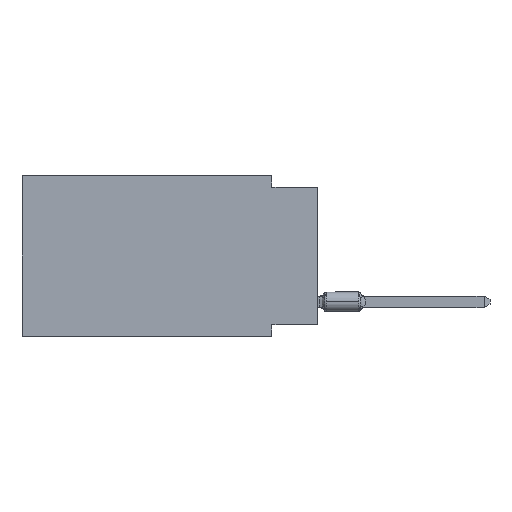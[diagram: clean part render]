
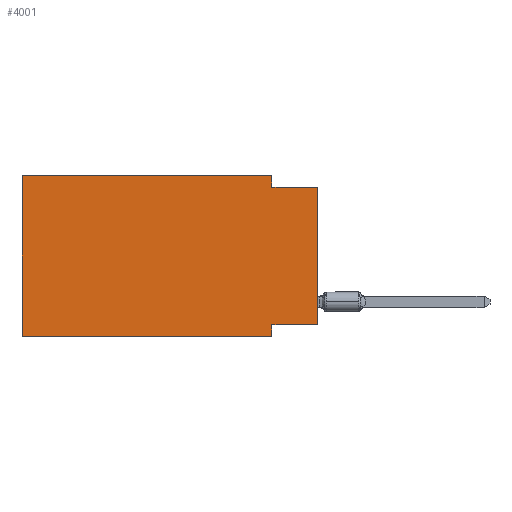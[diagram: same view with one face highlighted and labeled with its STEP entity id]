
A CAD part, left-side view. The second image highlights one B-rep face of the part: STEP entity #4001.
In plain terms, the highlighted planar face has unit normal (-1, 0, 0).
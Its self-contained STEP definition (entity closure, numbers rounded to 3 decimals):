
#301 = CARTESIAN_POINT ( 'NONE',  ( 0., 0., -8.255 ) ) ;
#351 = LINE ( 'NONE', #5917, #7434 ) ;
#478 = CARTESIAN_POINT ( 'NONE',  ( 0., 16.383, 0. ) ) ;
#701 = LINE ( 'NONE', #14898, #13395 ) ;
#754 = VECTOR ( 'NONE', #15659, 1000. ) ;
#1007 = CARTESIAN_POINT ( 'NONE',  ( 0., 16.383, 0. ) ) ;
#1133 = VECTOR ( 'NONE', #12843, 1000. ) ;
#1150 = DIRECTION ( 'NONE',  ( 0., -1., 0. ) ) ;
#1286 = CARTESIAN_POINT ( 'NONE',  ( 0., 0., -0.635 ) ) ;
#1605 = CARTESIAN_POINT ( 'NONE',  ( 0., 2.54, -8.255 ) ) ;
#1700 = CARTESIAN_POINT ( 'NONE',  ( 0., 2.54, -8.89 ) ) ;
#1791 = DIRECTION ( 'NONE',  ( 0., -1., 0. ) ) ;
#2219 = VECTOR ( 'NONE', #1791, 1000. ) ;
#2602 = ORIENTED_EDGE ( 'NONE', *, *, #8361, .T. ) ;
#2724 = VERTEX_POINT ( 'NONE', #1286 ) ;
#3174 = DIRECTION ( 'NONE',  ( 0., 0., -1. ) ) ;
#3936 = VERTEX_POINT ( 'NONE', #14567 ) ;
#4001 = ADVANCED_FACE ( 'NONE', ( #13475 ), #10969, .F. ) ;
#4195 = ORIENTED_EDGE ( 'NONE', *, *, #8038, .F. ) ;
#4328 = VECTOR ( 'NONE', #1150, 1000. ) ;
#4363 = VERTEX_POINT ( 'NONE', #7574 ) ;
#4878 = ORIENTED_EDGE ( 'NONE', *, *, #8454, .F. ) ;
#5448 = VERTEX_POINT ( 'NONE', #8599 ) ;
#5638 = LINE ( 'NONE', #8760, #2219 ) ;
#5833 = VERTEX_POINT ( 'NONE', #1605 ) ;
#5917 = CARTESIAN_POINT ( 'NONE',  ( 0., 16.383, 0. ) ) ;
#5918 = EDGE_LOOP ( 'NONE', ( #13003, #4195, #8770, #11957, #4878, #2602, #10950, #8723 ) ) ;
#6533 = LINE ( 'NONE', #10759, #4328 ) ;
#7222 = EDGE_CURVE ( 'NONE', #3936, #5833, #9633, .T. ) ;
#7434 = VECTOR ( 'NONE', #11496, 1000. ) ;
#7574 = CARTESIAN_POINT ( 'NONE',  ( 0., 2.54, 0. ) ) ;
#8038 = EDGE_CURVE ( 'NONE', #9749, #2724, #5638, .T. ) ;
#8113 = VERTEX_POINT ( 'NONE', #15612 ) ;
#8202 = VECTOR ( 'NONE', #12133, 1000. ) ;
#8361 = EDGE_CURVE ( 'NONE', #8113, #10505, #6533, .T. ) ;
#8454 = EDGE_CURVE ( 'NONE', #8113, #5448, #14306, .T. ) ;
#8599 = CARTESIAN_POINT ( 'NONE',  ( 0., 16.383, 0. ) ) ;
#8723 = ORIENTED_EDGE ( 'NONE', *, *, #7222, .F. ) ;
#8760 = CARTESIAN_POINT ( 'NONE',  ( 0., 0., -0.635 ) ) ;
#8770 = ORIENTED_EDGE ( 'NONE', *, *, #16653, .F. ) ;
#8938 = DIRECTION ( 'NONE',  ( 0., 0., 1. ) ) ;
#9289 = EDGE_CURVE ( 'NONE', #5448, #4363, #351, .T. ) ;
#9314 = EDGE_CURVE ( 'NONE', #5833, #10505, #15708, .T. ) ;
#9479 = CARTESIAN_POINT ( 'NONE',  ( 0., 2.54, 0. ) ) ;
#9633 = LINE ( 'NONE', #301, #754 ) ;
#9749 = VERTEX_POINT ( 'NONE', #10288 ) ;
#10288 = CARTESIAN_POINT ( 'NONE',  ( 0., 2.54, -0.635 ) ) ;
#10505 = VERTEX_POINT ( 'NONE', #1700 ) ;
#10759 = CARTESIAN_POINT ( 'NONE',  ( 0., 16.383, -8.89 ) ) ;
#10950 = ORIENTED_EDGE ( 'NONE', *, *, #9314, .F. ) ;
#10969 = PLANE ( 'NONE',  #17941 ) ;
#11226 = CARTESIAN_POINT ( 'NONE',  ( 0., 2.54, -8.89 ) ) ;
#11496 = DIRECTION ( 'NONE',  ( 0., -1., 0. ) ) ;
#11836 = EDGE_CURVE ( 'NONE', #3936, #2724, #701, .T. ) ;
#11957 = ORIENTED_EDGE ( 'NONE', *, *, #9289, .F. ) ;
#12133 = DIRECTION ( 'NONE',  ( 0., 0., -1. ) ) ;
#12355 = DIRECTION ( 'NONE',  ( 0., 0., -1. ) ) ;
#12843 = DIRECTION ( 'NONE',  ( 0., 0., 1. ) ) ;
#13003 = ORIENTED_EDGE ( 'NONE', *, *, #11836, .T. ) ;
#13395 = VECTOR ( 'NONE', #8938, 1000. ) ;
#13475 = FACE_OUTER_BOUND ( 'NONE', #5918, .T. ) ;
#13710 = LINE ( 'NONE', #9479, #8202 ) ;
#14306 = LINE ( 'NONE', #478, #1133 ) ;
#14567 = CARTESIAN_POINT ( 'NONE',  ( 0., 0., -8.255 ) ) ;
#14748 = DIRECTION ( 'NONE',  ( 1., 0., 0. ) ) ;
#14898 = CARTESIAN_POINT ( 'NONE',  ( 0., 0., 0. ) ) ;
#15612 = CARTESIAN_POINT ( 'NONE',  ( 0., 16.383, -8.89 ) ) ;
#15659 = DIRECTION ( 'NONE',  ( 0., 1., 0. ) ) ;
#15708 = LINE ( 'NONE', #11226, #17692 ) ;
#16653 = EDGE_CURVE ( 'NONE', #4363, #9749, #13710, .T. ) ;
#17692 = VECTOR ( 'NONE', #3174, 1000. ) ;
#17941 = AXIS2_PLACEMENT_3D ( 'NONE', #1007, #14748, #12355 ) ;
